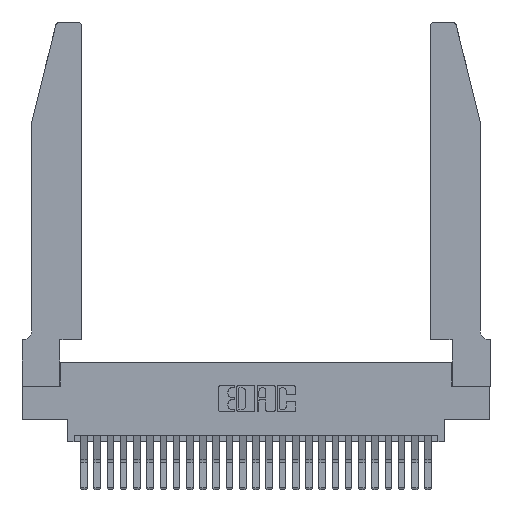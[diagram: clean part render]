
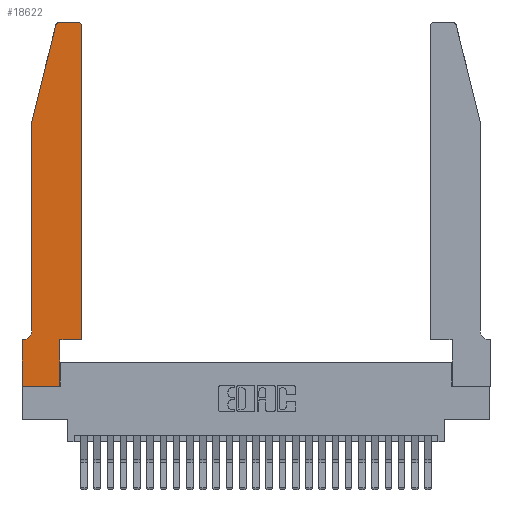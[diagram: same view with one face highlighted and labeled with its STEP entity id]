
A CAD part, top view. The second image highlights one B-rep face of the part: STEP entity #18622.
In plain terms, the highlighted planar face has unit normal (0, 0, 1).
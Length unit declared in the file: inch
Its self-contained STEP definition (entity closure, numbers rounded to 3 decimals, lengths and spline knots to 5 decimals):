
#484 = VERTEX_POINT ( 'NONE', #26289 ) ;
#927 = ORIENTED_EDGE ( 'NONE', *, *, #3082, .T. ) ;
#988 = EDGE_CURVE ( 'NONE', #20504, #27962, #22728, .T. ) ;
#1872 = VERTEX_POINT ( 'NONE', #3589 ) ;
#1883 = ORIENTED_EDGE ( 'NONE', *, *, #16227, .T. ) ;
#3082 = EDGE_CURVE ( 'NONE', #23476, #11150, #16699, .T. ) ;
#3233 = ORIENTED_EDGE ( 'NONE', *, *, #19721, .T. ) ;
#3271 = CARTESIAN_POINT ( 'NONE',  ( 0.4505, 0.35, 0.37 ) ) ;
#3471 = LINE ( 'NONE', #13111, #15203 ) ;
#3589 = CARTESIAN_POINT ( 'NONE',  ( 0.0055, 0.35, 0.37 ) ) ;
#3984 = LINE ( 'NONE', #3271, #4701 ) ;
#3994 = DIRECTION ( 'NONE',  ( -1., 0., 0. ) ) ;
#4259 = VECTOR ( 'NONE', #3994, 39.37008 ) ;
#4701 = VECTOR ( 'NONE', #9980, 39.37008 ) ;
#4833 = ORIENTED_EDGE ( 'NONE', *, *, #988, .T. ) ;
#5041 = CARTESIAN_POINT ( 'NONE',  ( 0., 0.35, 0.37 ) ) ;
#5113 = CARTESIAN_POINT ( 'NONE',  ( 0.0755, 0.42, 0.37 ) ) ;
#5318 = LINE ( 'NONE', #13384, #27452 ) ;
#6468 = LINE ( 'NONE', #11502, #11607 ) ;
#7073 = ORIENTED_EDGE ( 'NONE', *, *, #10112, .T. ) ;
#7340 = DIRECTION ( 'NONE',  ( 1., 0., 0. ) ) ;
#7857 = EDGE_CURVE ( 'NONE', #484, #20530, #10956, .T. ) ;
#8055 = DIRECTION ( 'NONE',  ( -1., 0., 0. ) ) ;
#8239 = EDGE_CURVE ( 'NONE', #17258, #23714, #13969, .T. ) ;
#8290 = CARTESIAN_POINT ( 'NONE',  ( 0.25487, 2.72718, 0.37 ) ) ;
#8635 = VECTOR ( 'NONE', #26932, 39.37008 ) ;
#8740 = CIRCLE ( 'NONE', #12747, 0.07 ) ;
#8756 = CARTESIAN_POINT ( 'NONE',  ( 0.2865, 0.35, 0.37 ) ) ;
#9695 = VERTEX_POINT ( 'NONE', #5113 ) ;
#9747 = CARTESIAN_POINT ( 'NONE',  ( 0.284, 2.72, 0.37 ) ) ;
#9980 = DIRECTION ( 'NONE',  ( 1., 0., 0. ) ) ;
#10112 = EDGE_CURVE ( 'NONE', #20530, #27131, #3471, .T. ) ;
#10360 = EDGE_CURVE ( 'NONE', #1872, #23476, #25417, .T. ) ;
#10663 = CARTESIAN_POINT ( 'NONE',  ( 0.2865, 0.35, 0.37 ) ) ;
#10922 = ORIENTED_EDGE ( 'NONE', *, *, #7857, .T. ) ;
#10956 = CIRCLE ( 'NONE', #27727, 0.03 ) ;
#11150 = VERTEX_POINT ( 'NONE', #17048 ) ;
#11502 = CARTESIAN_POINT ( 'NONE',  ( 0.0755, 2., 0.37 ) ) ;
#11607 = VECTOR ( 'NONE', #19980, 39.37008 ) ;
#11694 = CARTESIAN_POINT ( 'NONE',  ( 0.4205, 2.75, 0.37 ) ) ;
#11713 = DIRECTION ( 'NONE',  ( 0., -1., 0. ) ) ;
#11904 = DIRECTION ( 'NONE',  ( 1., 0., 0. ) ) ;
#12082 = CARTESIAN_POINT ( 'NONE',  ( 0.0755, 2., 0.37 ) ) ;
#12331 = CARTESIAN_POINT ( 'NONE',  ( 0.0755, 0.35, 0.37 ) ) ;
#12747 = AXIS2_PLACEMENT_3D ( 'NONE', #26021, #13381, #28143 ) ;
#13111 = CARTESIAN_POINT ( 'NONE',  ( 0.0755, 2., 0.37 ) ) ;
#13119 = DIRECTION ( 'NONE',  ( 0., 1., 0. ) ) ;
#13321 = EDGE_CURVE ( 'NONE', #25514, #20504, #22005, .T. ) ;
#13381 = DIRECTION ( 'NONE',  ( 0., 0., -1. ) ) ;
#13384 = CARTESIAN_POINT ( 'NONE',  ( 0., 0., 0.37 ) ) ;
#13514 = VECTOR ( 'NONE', #8055, 39.37008 ) ;
#13716 = PLANE ( 'NONE',  #23529 ) ;
#13969 = LINE ( 'NONE', #8756, #24556 ) ;
#14292 = CARTESIAN_POINT ( 'NONE',  ( 0.4505, 0.35, 0.37 ) ) ;
#14390 = EDGE_CURVE ( 'NONE', #27131, #9695, #6468, .T. ) ;
#14904 = ORIENTED_EDGE ( 'NONE', *, *, #14390, .T. ) ;
#15203 = VECTOR ( 'NONE', #15264, 39.37008 ) ;
#15264 = DIRECTION ( 'NONE',  ( -0.239, -0.971, 0. ) ) ;
#15537 = DIRECTION ( 'NONE',  ( 1., 0., 0. ) ) ;
#15784 = AXIS2_PLACEMENT_3D ( 'NONE', #16354, #16259, #16182 ) ;
#15921 = LINE ( 'NONE', #19244, #4259 ) ;
#16039 = VECTOR ( 'NONE', #11713, 39.37008 ) ;
#16182 = DIRECTION ( 'NONE',  ( 1., 0., 0. ) ) ;
#16227 = EDGE_CURVE ( 'NONE', #11150, #17258, #5318, .T. ) ;
#16259 = DIRECTION ( 'NONE',  ( 0., 0., 1. ) ) ;
#16354 = CARTESIAN_POINT ( 'NONE',  ( 0.4205, 2.72, 0.37 ) ) ;
#16389 = CARTESIAN_POINT ( 'NONE',  ( 0., 0.35, 0.37 ) ) ;
#16699 = LINE ( 'NONE', #20368, #16039 ) ;
#17048 = CARTESIAN_POINT ( 'NONE',  ( 0., 0., 0.37 ) ) ;
#17258 = VERTEX_POINT ( 'NONE', #27534 ) ;
#17957 = ORIENTED_EDGE ( 'NONE', *, *, #10360, .T. ) ;
#18622 = ADVANCED_FACE ( 'NONE', ( #19759 ), #13716, .T. ) ;
#19244 = CARTESIAN_POINT ( 'NONE',  ( 0.2605, 2.75, 0.37 ) ) ;
#19721 = EDGE_CURVE ( 'NONE', #23714, #25514, #3984, .T. ) ;
#19759 = FACE_OUTER_BOUND ( 'NONE', #24222, .T. ) ;
#19980 = DIRECTION ( 'NONE',  ( 0., -1., 0. ) ) ;
#20219 = DIRECTION ( 'NONE',  ( 0., 0., 1. ) ) ;
#20368 = CARTESIAN_POINT ( 'NONE',  ( 0., 0., 0.37 ) ) ;
#20504 = VERTEX_POINT ( 'NONE', #27173 ) ;
#20530 = VERTEX_POINT ( 'NONE', #8290 ) ;
#20642 = ORIENTED_EDGE ( 'NONE', *, *, #21282, .T. ) ;
#21282 = EDGE_CURVE ( 'NONE', #27962, #484, #15921, .T. ) ;
#22005 = LINE ( 'NONE', #14292, #8635 ) ;
#22728 = CIRCLE ( 'NONE', #15784, 0.03 ) ;
#23476 = VERTEX_POINT ( 'NONE', #16389 ) ;
#23529 = AXIS2_PLACEMENT_3D ( 'NONE', #5041, #20219, #7340 ) ;
#23714 = VERTEX_POINT ( 'NONE', #10663 ) ;
#23844 = EDGE_CURVE ( 'NONE', #9695, #1872, #8740, .T. ) ;
#23959 = CARTESIAN_POINT ( 'NONE',  ( 0.4505, 0.35, 0.37 ) ) ;
#24222 = EDGE_LOOP ( 'NONE', ( #20642, #10922, #7073, #14904, #27917, #17957, #927, #1883, #25059, #3233, #26697, #4833 ) ) ;
#24556 = VECTOR ( 'NONE', #13119, 39.37008 ) ;
#24619 = DIRECTION ( 'NONE',  ( 0., 0., 1. ) ) ;
#25059 = ORIENTED_EDGE ( 'NONE', *, *, #8239, .T. ) ;
#25417 = LINE ( 'NONE', #12331, #13514 ) ;
#25514 = VERTEX_POINT ( 'NONE', #23959 ) ;
#26021 = CARTESIAN_POINT ( 'NONE',  ( 0.0055, 0.42, 0.37 ) ) ;
#26289 = CARTESIAN_POINT ( 'NONE',  ( 0.284, 2.75, 0.37 ) ) ;
#26697 = ORIENTED_EDGE ( 'NONE', *, *, #13321, .T. ) ;
#26932 = DIRECTION ( 'NONE',  ( 0., 1., 0. ) ) ;
#27131 = VERTEX_POINT ( 'NONE', #12082 ) ;
#27173 = CARTESIAN_POINT ( 'NONE',  ( 0.4505, 2.72, 0.37 ) ) ;
#27452 = VECTOR ( 'NONE', #15537, 39.37008 ) ;
#27534 = CARTESIAN_POINT ( 'NONE',  ( 0.2865, 0., 0.37 ) ) ;
#27727 = AXIS2_PLACEMENT_3D ( 'NONE', #9747, #24619, #11904 ) ;
#27917 = ORIENTED_EDGE ( 'NONE', *, *, #23844, .T. ) ;
#27962 = VERTEX_POINT ( 'NONE', #11694 ) ;
#28143 = DIRECTION ( 'NONE',  ( -1., 0., 0. ) ) ;
